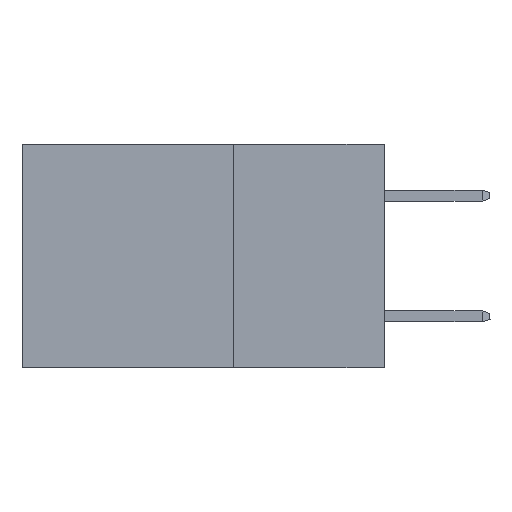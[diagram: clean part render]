
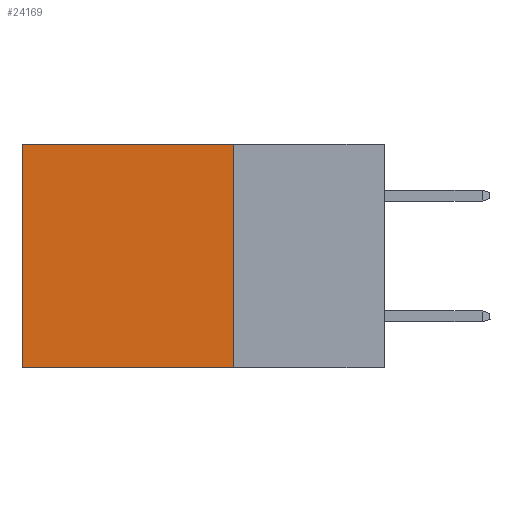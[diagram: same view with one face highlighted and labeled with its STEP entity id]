
A CAD part, left-side view. The second image highlights one B-rep face of the part: STEP entity #24169.
In plain terms, the highlighted planar face has unit normal (-1, 0, 0).
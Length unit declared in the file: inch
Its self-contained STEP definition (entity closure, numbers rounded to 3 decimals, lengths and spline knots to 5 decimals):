
#75 = DIRECTION ( 'NONE',  ( 0., 0., -1. ) ) ;
#2182 = CARTESIAN_POINT ( 'NONE',  ( 0.2615, 0.25, -0.37 ) ) ;
#2790 = PLANE ( 'NONE',  #25772 ) ;
#3347 = CARTESIAN_POINT ( 'NONE',  ( 0.2615, 0.25, -0.37 ) ) ;
#3935 = EDGE_CURVE ( 'NONE', #16708, #5224, #19488, .T. ) ;
#4239 = LINE ( 'NONE', #14404, #9692 ) ;
#4250 = DIRECTION ( 'NONE',  ( 0., 0., -1. ) ) ;
#4265 = VECTOR ( 'NONE', #19251, 39.37008 ) ;
#5224 = VERTEX_POINT ( 'NONE', #10463 ) ;
#7625 = ORIENTED_EDGE ( 'NONE', *, *, #16587, .T. ) ;
#7694 = FACE_OUTER_BOUND ( 'NONE', #24755, .T. ) ;
#8967 = DIRECTION ( 'NONE',  ( 0., 0., -1. ) ) ;
#9356 = EDGE_CURVE ( 'NONE', #5224, #19006, #15603, .T. ) ;
#9692 = VECTOR ( 'NONE', #75, 39.37008 ) ;
#10463 = CARTESIAN_POINT ( 'NONE',  ( 0.2615, 0.25, -0.37 ) ) ;
#11250 = ORIENTED_EDGE ( 'NONE', *, *, #3935, .F. ) ;
#12165 = ORIENTED_EDGE ( 'NONE', *, *, #9356, .F. ) ;
#14144 = VECTOR ( 'NONE', #4250, 39.37008 ) ;
#14150 = VERTEX_POINT ( 'NONE', #16828 ) ;
#14404 = CARTESIAN_POINT ( 'NONE',  ( 0.2615, 0.6, -0.37 ) ) ;
#14968 = VECTOR ( 'NONE', #21607, 39.37008 ) ;
#15187 = ORIENTED_EDGE ( 'NONE', *, *, #17020, .T. ) ;
#15603 = LINE ( 'NONE', #3347, #14968 ) ;
#16587 = EDGE_CURVE ( 'NONE', #16708, #14150, #21084, .T. ) ;
#16708 = VERTEX_POINT ( 'NONE', #17591 ) ;
#16828 = CARTESIAN_POINT ( 'NONE',  ( 0.2615, 0.6, 0. ) ) ;
#16947 = CARTESIAN_POINT ( 'NONE',  ( 0.2615, 0.25, -0.37 ) ) ;
#17020 = EDGE_CURVE ( 'NONE', #14150, #19006, #4239, .T. ) ;
#17256 = CARTESIAN_POINT ( 'NONE',  ( 0.2615, 0.25, 0. ) ) ;
#17591 = CARTESIAN_POINT ( 'NONE',  ( 0.2615, 0.25, 0. ) ) ;
#18788 = CARTESIAN_POINT ( 'NONE',  ( 0.2615, 0.6, -0.37 ) ) ;
#19006 = VERTEX_POINT ( 'NONE', #18788 ) ;
#19251 = DIRECTION ( 'NONE',  ( 0., 1., 0. ) ) ;
#19488 = LINE ( 'NONE', #2182, #14144 ) ;
#21065 = DIRECTION ( 'NONE',  ( 1., 0., 0. ) ) ;
#21084 = LINE ( 'NONE', #17256, #4265 ) ;
#21607 = DIRECTION ( 'NONE',  ( 0., 1., 0. ) ) ;
#24169 = ADVANCED_FACE ( 'NONE', ( #7694 ), #2790, .F. ) ;
#24755 = EDGE_LOOP ( 'NONE', ( #15187, #12165, #11250, #7625 ) ) ;
#25772 = AXIS2_PLACEMENT_3D ( 'NONE', #16947, #21065, #8967 ) ;
